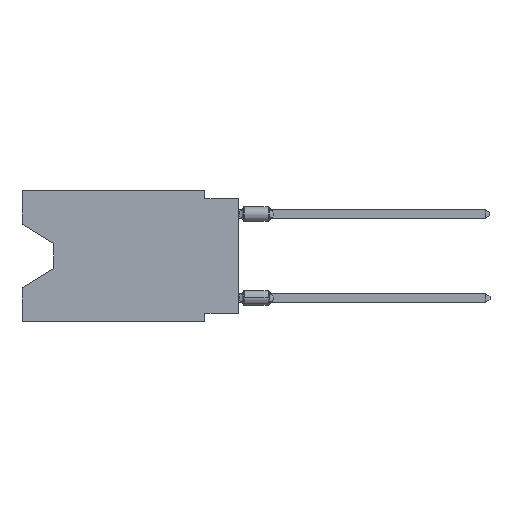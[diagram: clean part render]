
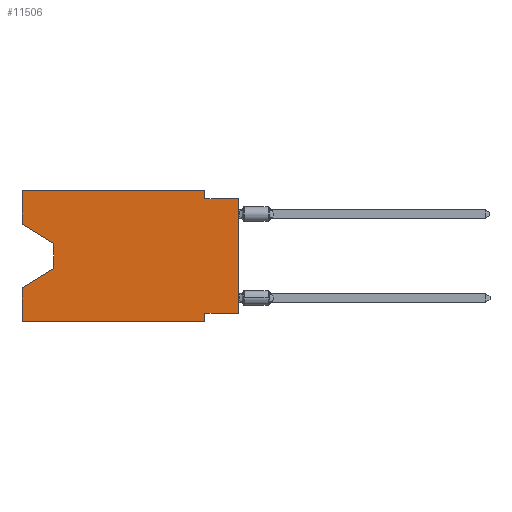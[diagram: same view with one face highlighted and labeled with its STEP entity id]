
A CAD part, left-side view. The second image highlights one B-rep face of the part: STEP entity #11506.
In plain terms, the highlighted planar face has unit normal (-1, 0, 0).
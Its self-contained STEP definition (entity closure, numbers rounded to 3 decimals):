
#620 = VECTOR ( 'NONE', #27207, 1000. ) ;
#697 = VECTOR ( 'NONE', #28837, 1000. ) ;
#789 = CARTESIAN_POINT ( 'NONE',  ( 0., 13.97, -4.013 ) ) ;
#994 = CARTESIAN_POINT ( 'NONE',  ( 0., 16.383, 0. ) ) ;
#1390 = CARTESIAN_POINT ( 'NONE',  ( 0., 13.97, -4.013 ) ) ;
#1880 = VERTEX_POINT ( 'NONE', #26699 ) ;
#1905 = DIRECTION ( 'NONE',  ( 0., -1., 0. ) ) ;
#2086 = VECTOR ( 'NONE', #2558, 1000. ) ;
#2558 = DIRECTION ( 'NONE',  ( 0., -1., 0. ) ) ;
#2659 = DIRECTION ( 'NONE',  ( 0., 0., 1. ) ) ;
#2768 = EDGE_CURVE ( 'NONE', #4480, #31043, #17372, .T. ) ;
#3200 = CARTESIAN_POINT ( 'NONE',  ( 0., 16.383, 0. ) ) ;
#3234 = LINE ( 'NONE', #13172, #25020 ) ;
#3385 = DIRECTION ( 'NONE',  ( 0., -1., 0. ) ) ;
#3517 = EDGE_CURVE ( 'NONE', #21924, #18917, #21995, .T. ) ;
#3865 = EDGE_CURVE ( 'NONE', #18248, #29621, #24032, .T. ) ;
#4279 = CARTESIAN_POINT ( 'NONE',  ( 0., 16.383, 0. ) ) ;
#4344 = VECTOR ( 'NONE', #1905, 1000. ) ;
#4480 = VERTEX_POINT ( 'NONE', #1390 ) ;
#4659 = VECTOR ( 'NONE', #9938, 1000. ) ;
#4992 = VERTEX_POINT ( 'NONE', #20452 ) ;
#5103 = CARTESIAN_POINT ( 'NONE',  ( 0., 2.54, -9.906 ) ) ;
#5249 = CARTESIAN_POINT ( 'NONE',  ( 0., 2.54, -0.635 ) ) ;
#5702 = LINE ( 'NONE', #20383, #27157 ) ;
#6167 = FACE_OUTER_BOUND ( 'NONE', #19700, .T. ) ;
#6735 = ORIENTED_EDGE ( 'NONE', *, *, #20499, .F. ) ;
#7253 = LINE ( 'NONE', #28430, #19176 ) ;
#7406 = DIRECTION ( 'NONE',  ( 0., -0.855, -0.519 ) ) ;
#7637 = LINE ( 'NONE', #22021, #697 ) ;
#7645 = CARTESIAN_POINT ( 'NONE',  ( 0., 0., -0.635 ) ) ;
#7660 = DIRECTION ( 'NONE',  ( 0., 0.855, -0.519 ) ) ;
#7999 = VECTOR ( 'NONE', #29542, 1000. ) ;
#8094 = EDGE_CURVE ( 'NONE', #18917, #1880, #18791, .T. ) ;
#8119 = ORIENTED_EDGE ( 'NONE', *, *, #8094, .F. ) ;
#9140 = ORIENTED_EDGE ( 'NONE', *, *, #20592, .F. ) ;
#9938 = DIRECTION ( 'NONE',  ( 0., 0., -1. ) ) ;
#10106 = DIRECTION ( 'NONE',  ( 0., 0., 1. ) ) ;
#10120 = AXIS2_PLACEMENT_3D ( 'NONE', #4279, #22891, #28274 ) ;
#11382 = EDGE_CURVE ( 'NONE', #14192, #4992, #15021, .T. ) ;
#11506 = ADVANCED_FACE ( 'NONE', ( #6167 ), #21018, .F. ) ;
#12073 = CARTESIAN_POINT ( 'NONE',  ( 0., 16.383, -7.36 ) ) ;
#12231 = EDGE_CURVE ( 'NONE', #31043, #13638, #17160, .T. ) ;
#12958 = LINE ( 'NONE', #20223, #7999 ) ;
#13172 = CARTESIAN_POINT ( 'NONE',  ( 0., 16.383, 0. ) ) ;
#13638 = VERTEX_POINT ( 'NONE', #12073 ) ;
#14121 = EDGE_CURVE ( 'NONE', #23393, #4992, #29292, .T. ) ;
#14192 = VERTEX_POINT ( 'NONE', #30221 ) ;
#15021 = LINE ( 'NONE', #17846, #28320 ) ;
#15195 = EDGE_CURVE ( 'NONE', #18248, #13638, #3234, .T. ) ;
#15494 = DIRECTION ( 'NONE',  ( 0., 0., -1. ) ) ;
#15817 = VECTOR ( 'NONE', #7660, 1000. ) ;
#15872 = ORIENTED_EDGE ( 'NONE', *, *, #14121, .F. ) ;
#16487 = CARTESIAN_POINT ( 'NONE',  ( 0., 16.383, -2.546 ) ) ;
#17160 = LINE ( 'NONE', #26639, #15817 ) ;
#17372 = LINE ( 'NONE', #789, #4659 ) ;
#17846 = CARTESIAN_POINT ( 'NONE',  ( 0., 0., 0. ) ) ;
#18248 = VERTEX_POINT ( 'NONE', #25431 ) ;
#18497 = ORIENTED_EDGE ( 'NONE', *, *, #3865, .T. ) ;
#18791 = LINE ( 'NONE', #28271, #4344 ) ;
#18917 = VERTEX_POINT ( 'NONE', #994 ) ;
#19176 = VECTOR ( 'NONE', #7406, 1000. ) ;
#19621 = VERTEX_POINT ( 'NONE', #28581 ) ;
#19700 = EDGE_LOOP ( 'NONE', ( #26048, #30543, #21743, #27437, #18497, #6735, #23637, #22528, #15872, #9140, #8119, #20030 ) ) ;
#20030 = ORIENTED_EDGE ( 'NONE', *, *, #3517, .F. ) ;
#20223 = CARTESIAN_POINT ( 'NONE',  ( 0., 2.54, 0. ) ) ;
#20383 = CARTESIAN_POINT ( 'NONE',  ( 0., 2.54, -9.906 ) ) ;
#20452 = CARTESIAN_POINT ( 'NONE',  ( 0., 0., -0.635 ) ) ;
#20499 = EDGE_CURVE ( 'NONE', #19621, #29621, #5702, .T. ) ;
#20592 = EDGE_CURVE ( 'NONE', #1880, #23393, #12958, .T. ) ;
#21018 = PLANE ( 'NONE',  #10120 ) ;
#21661 = CARTESIAN_POINT ( 'NONE',  ( 0., 16.383, -9.906 ) ) ;
#21743 = ORIENTED_EDGE ( 'NONE', *, *, #12231, .T. ) ;
#21924 = VERTEX_POINT ( 'NONE', #16487 ) ;
#21995 = LINE ( 'NONE', #3200, #620 ) ;
#22021 = CARTESIAN_POINT ( 'NONE',  ( 0., 0., -9.271 ) ) ;
#22528 = ORIENTED_EDGE ( 'NONE', *, *, #11382, .T. ) ;
#22891 = DIRECTION ( 'NONE',  ( 1., 0., 0. ) ) ;
#23393 = VERTEX_POINT ( 'NONE', #5249 ) ;
#23637 = ORIENTED_EDGE ( 'NONE', *, *, #30443, .F. ) ;
#24032 = LINE ( 'NONE', #21661, #2086 ) ;
#24518 = CARTESIAN_POINT ( 'NONE',  ( 0., 13.97, -5.893 ) ) ;
#24939 = VECTOR ( 'NONE', #3385, 1000. ) ;
#25020 = VECTOR ( 'NONE', #2659, 1000. ) ;
#25431 = CARTESIAN_POINT ( 'NONE',  ( 0., 16.383, -9.906 ) ) ;
#26048 = ORIENTED_EDGE ( 'NONE', *, *, #27516, .T. ) ;
#26639 = CARTESIAN_POINT ( 'NONE',  ( 0., 13.97, -5.893 ) ) ;
#26699 = CARTESIAN_POINT ( 'NONE',  ( 0., 2.54, 0. ) ) ;
#27157 = VECTOR ( 'NONE', #15494, 1000. ) ;
#27207 = DIRECTION ( 'NONE',  ( 0., 0., 1. ) ) ;
#27437 = ORIENTED_EDGE ( 'NONE', *, *, #15195, .F. ) ;
#27516 = EDGE_CURVE ( 'NONE', #21924, #4480, #7253, .T. ) ;
#28271 = CARTESIAN_POINT ( 'NONE',  ( 0., 16.383, 0. ) ) ;
#28274 = DIRECTION ( 'NONE',  ( 0., 0., -1. ) ) ;
#28320 = VECTOR ( 'NONE', #10106, 1000. ) ;
#28430 = CARTESIAN_POINT ( 'NONE',  ( 0., 16.383, -2.546 ) ) ;
#28581 = CARTESIAN_POINT ( 'NONE',  ( 0., 2.54, -9.271 ) ) ;
#28837 = DIRECTION ( 'NONE',  ( 0., 1., 0. ) ) ;
#29292 = LINE ( 'NONE', #7645, #24939 ) ;
#29542 = DIRECTION ( 'NONE',  ( 0., 0., -1. ) ) ;
#29621 = VERTEX_POINT ( 'NONE', #5103 ) ;
#30221 = CARTESIAN_POINT ( 'NONE',  ( 0., 0., -9.271 ) ) ;
#30443 = EDGE_CURVE ( 'NONE', #14192, #19621, #7637, .T. ) ;
#30543 = ORIENTED_EDGE ( 'NONE', *, *, #2768, .T. ) ;
#31043 = VERTEX_POINT ( 'NONE', #24518 ) ;
